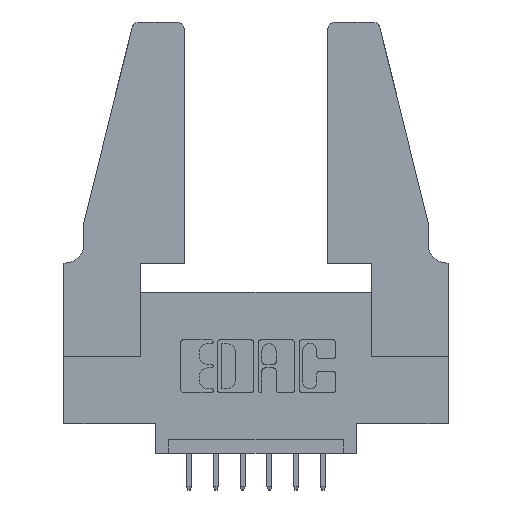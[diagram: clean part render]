
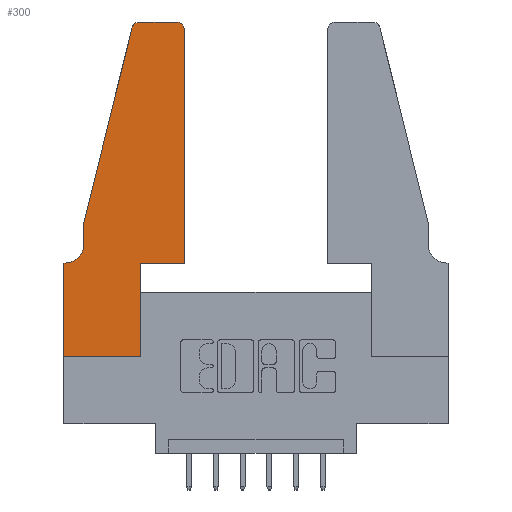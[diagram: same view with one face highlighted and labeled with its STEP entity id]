
A CAD part, top view. The second image highlights one B-rep face of the part: STEP entity #300.
In plain terms, the highlighted planar face has unit normal (0, 0, 1).
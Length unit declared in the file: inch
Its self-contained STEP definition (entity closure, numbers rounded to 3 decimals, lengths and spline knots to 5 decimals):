
#84 = FACE_OUTER_BOUND ( 'NONE', #1701, .T. ) ;
#161 = ORIENTED_EDGE ( 'NONE', *, *, #2911, .T. ) ;
#300 = ADVANCED_FACE ( 'NONE', ( #84 ), #11146, .T. ) ;
#352 = CIRCLE ( 'NONE', #6984, 0.03 ) ;
#399 = VERTEX_POINT ( 'NONE', #10193 ) ;
#406 = VECTOR ( 'NONE', #9704, 39.37008 ) ;
#605 = LINE ( 'NONE', #10768, #406 ) ;
#771 = AXIS2_PLACEMENT_3D ( 'NONE', #10401, #11176, #2147 ) ;
#806 = VERTEX_POINT ( 'NONE', #1854 ) ;
#910 = ORIENTED_EDGE ( 'NONE', *, *, #3648, .T. ) ;
#1053 = LINE ( 'NONE', #10148, #8186 ) ;
#1069 = EDGE_CURVE ( 'NONE', #11479, #8435, #605, .T. ) ;
#1091 = LINE ( 'NONE', #3118, #1972 ) ;
#1151 = CARTESIAN_POINT ( 'NONE',  ( 0.0755, 0.5, 0.37 ) ) ;
#1215 = CARTESIAN_POINT ( 'NONE',  ( 0.2605, 1.25, 0.37 ) ) ;
#1334 = EDGE_CURVE ( 'NONE', #10206, #2501, #7230, .T. ) ;
#1701 = EDGE_LOOP ( 'NONE', ( #6340, #910, #161, #8053, #6918, #3595, #3008, #4183, #7042, #10715, #10038, #2031 ) ) ;
#1854 = CARTESIAN_POINT ( 'NONE',  ( 0.2865, 0., 0.37 ) ) ;
#1972 = VECTOR ( 'NONE', #11135, 39.37008 ) ;
#2031 = ORIENTED_EDGE ( 'NONE', *, *, #1334, .T. ) ;
#2052 = VERTEX_POINT ( 'NONE', #5866 ) ;
#2147 = DIRECTION ( 'NONE',  ( 1., 0., 0. ) ) ;
#2501 = VERTEX_POINT ( 'NONE', #3013 ) ;
#2653 = CARTESIAN_POINT ( 'NONE',  ( 0.25487, 1.22718, 0.37 ) ) ;
#2871 = EDGE_CURVE ( 'NONE', #806, #6343, #5657, .T. ) ;
#2911 = EDGE_CURVE ( 'NONE', #3997, #5172, #9303, .T. ) ;
#2938 = EDGE_CURVE ( 'NONE', #2501, #11485, #11194, .T. ) ;
#3008 = ORIENTED_EDGE ( 'NONE', *, *, #1069, .T. ) ;
#3013 = CARTESIAN_POINT ( 'NONE',  ( 0.4205, 1.25, 0.37 ) ) ;
#3093 = CIRCLE ( 'NONE', #9133, 0.07 ) ;
#3118 = CARTESIAN_POINT ( 'NONE',  ( 0., 0., 0.37 ) ) ;
#3255 = CARTESIAN_POINT ( 'NONE',  ( 0.0755, 0.5, 0.37 ) ) ;
#3595 = ORIENTED_EDGE ( 'NONE', *, *, #9669, .T. ) ;
#3623 = LINE ( 'NONE', #8269, #5541 ) ;
#3648 = EDGE_CURVE ( 'NONE', #11485, #3997, #352, .T. ) ;
#3760 = DIRECTION ( 'NONE',  ( 0., 1., 0. ) ) ;
#3890 = DIRECTION ( 'NONE',  ( 0., 0., -1. ) ) ;
#3997 = VERTEX_POINT ( 'NONE', #2653 ) ;
#4110 = CARTESIAN_POINT ( 'NONE',  ( 0.2865, 0.35, 0.37 ) ) ;
#4183 = ORIENTED_EDGE ( 'NONE', *, *, #11486, .T. ) ;
#4258 = DIRECTION ( 'NONE',  ( 0., -1., 0. ) ) ;
#4605 = CARTESIAN_POINT ( 'NONE',  ( 0., 0.35, 0.37 ) ) ;
#4817 = CARTESIAN_POINT ( 'NONE',  ( 0.4505, 0.35, 0.37 ) ) ;
#4933 = LINE ( 'NONE', #5878, #9545 ) ;
#5004 = VECTOR ( 'NONE', #11116, 39.37008 ) ;
#5172 = VERTEX_POINT ( 'NONE', #3255 ) ;
#5452 = VECTOR ( 'NONE', #9363, 39.37008 ) ;
#5541 = VECTOR ( 'NONE', #6539, 39.37008 ) ;
#5657 = LINE ( 'NONE', #7512, #10004 ) ;
#5800 = DIRECTION ( 'NONE',  ( 0., 1., 0. ) ) ;
#5865 = VERTEX_POINT ( 'NONE', #10844 ) ;
#5866 = CARTESIAN_POINT ( 'NONE',  ( 0.0055, 0.35, 0.37 ) ) ;
#5878 = CARTESIAN_POINT ( 'NONE',  ( 0.0755, 0.5, 0.37 ) ) ;
#6340 = ORIENTED_EDGE ( 'NONE', *, *, #2938, .T. ) ;
#6343 = VERTEX_POINT ( 'NONE', #4110 ) ;
#6539 = DIRECTION ( 'NONE',  ( -1., 0., 0. ) ) ;
#6566 = DIRECTION ( 'NONE',  ( -1., 0., 0. ) ) ;
#6580 = CARTESIAN_POINT ( 'NONE',  ( 0., 0., 0.37 ) ) ;
#6726 = AXIS2_PLACEMENT_3D ( 'NONE', #4605, #10136, #10907 ) ;
#6918 = ORIENTED_EDGE ( 'NONE', *, *, #7585, .T. ) ;
#6984 = AXIS2_PLACEMENT_3D ( 'NONE', #8082, #9695, #8812 ) ;
#7042 = ORIENTED_EDGE ( 'NONE', *, *, #2871, .T. ) ;
#7230 = CIRCLE ( 'NONE', #771, 0.03 ) ;
#7434 = LINE ( 'NONE', #4817, #5004 ) ;
#7512 = CARTESIAN_POINT ( 'NONE',  ( 0.2865, 0.35, 0.37 ) ) ;
#7585 = EDGE_CURVE ( 'NONE', #399, #2052, #3093, .T. ) ;
#8053 = ORIENTED_EDGE ( 'NONE', *, *, #9824, .T. ) ;
#8082 = CARTESIAN_POINT ( 'NONE',  ( 0.284, 1.22, 0.37 ) ) ;
#8186 = VECTOR ( 'NONE', #5800, 39.37008 ) ;
#8269 = CARTESIAN_POINT ( 'NONE',  ( 0.0755, 0.35, 0.37 ) ) ;
#8409 = DIRECTION ( 'NONE',  ( -0.239, -0.971, 0. ) ) ;
#8435 = VERTEX_POINT ( 'NONE', #6580 ) ;
#8449 = EDGE_CURVE ( 'NONE', #5865, #10206, #1053, .T. ) ;
#8812 = DIRECTION ( 'NONE',  ( 1., 0., 0. ) ) ;
#9133 = AXIS2_PLACEMENT_3D ( 'NONE', #10957, #3890, #6566 ) ;
#9303 = LINE ( 'NONE', #1151, #11708 ) ;
#9363 = DIRECTION ( 'NONE',  ( -1., 0., 0. ) ) ;
#9545 = VECTOR ( 'NONE', #4258, 39.37008 ) ;
#9669 = EDGE_CURVE ( 'NONE', #2052, #11479, #3623, .T. ) ;
#9695 = DIRECTION ( 'NONE',  ( 0., 0., 1. ) ) ;
#9704 = DIRECTION ( 'NONE',  ( 0., -1., 0. ) ) ;
#9824 = EDGE_CURVE ( 'NONE', #5172, #399, #4933, .T. ) ;
#10004 = VECTOR ( 'NONE', #3760, 39.37008 ) ;
#10038 = ORIENTED_EDGE ( 'NONE', *, *, #8449, .T. ) ;
#10125 = CARTESIAN_POINT ( 'NONE',  ( 0.284, 1.25, 0.37 ) ) ;
#10136 = DIRECTION ( 'NONE',  ( 0., 0., 1. ) ) ;
#10148 = CARTESIAN_POINT ( 'NONE',  ( 0.4505, 0.35, 0.37 ) ) ;
#10193 = CARTESIAN_POINT ( 'NONE',  ( 0.0755, 0.42, 0.37 ) ) ;
#10206 = VERTEX_POINT ( 'NONE', #11469 ) ;
#10369 = CARTESIAN_POINT ( 'NONE',  ( 0., 0.35, 0.37 ) ) ;
#10401 = CARTESIAN_POINT ( 'NONE',  ( 0.4205, 1.22, 0.37 ) ) ;
#10574 = EDGE_CURVE ( 'NONE', #6343, #5865, #7434, .T. ) ;
#10715 = ORIENTED_EDGE ( 'NONE', *, *, #10574, .T. ) ;
#10768 = CARTESIAN_POINT ( 'NONE',  ( 0., 0., 0.37 ) ) ;
#10844 = CARTESIAN_POINT ( 'NONE',  ( 0.4505, 0.35, 0.37 ) ) ;
#10907 = DIRECTION ( 'NONE',  ( 1., 0., 0. ) ) ;
#10957 = CARTESIAN_POINT ( 'NONE',  ( 0.0055, 0.42, 0.37 ) ) ;
#11116 = DIRECTION ( 'NONE',  ( 1., 0., 0. ) ) ;
#11135 = DIRECTION ( 'NONE',  ( 1., 0., 0. ) ) ;
#11146 = PLANE ( 'NONE',  #6726 ) ;
#11176 = DIRECTION ( 'NONE',  ( 0., 0., 1. ) ) ;
#11194 = LINE ( 'NONE', #1215, #5452 ) ;
#11469 = CARTESIAN_POINT ( 'NONE',  ( 0.4505, 1.22, 0.37 ) ) ;
#11479 = VERTEX_POINT ( 'NONE', #10369 ) ;
#11485 = VERTEX_POINT ( 'NONE', #10125 ) ;
#11486 = EDGE_CURVE ( 'NONE', #8435, #806, #1091, .T. ) ;
#11708 = VECTOR ( 'NONE', #8409, 39.37008 ) ;
